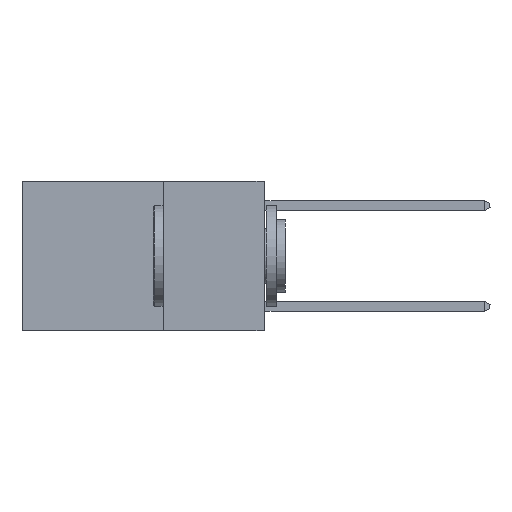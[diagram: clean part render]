
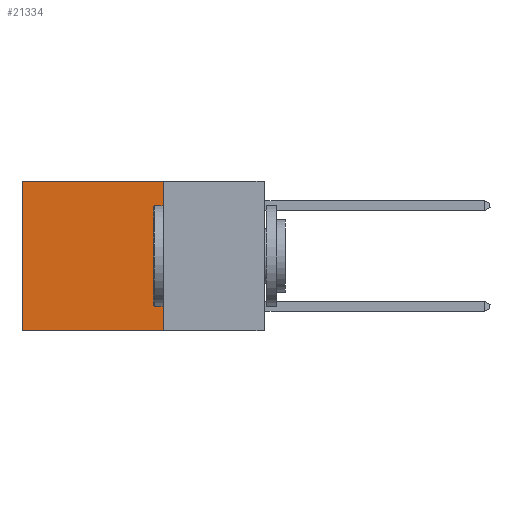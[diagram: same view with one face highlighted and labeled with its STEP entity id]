
A CAD part, left-side view. The second image highlights one B-rep face of the part: STEP entity #21334.
In plain terms, the highlighted planar face has unit normal (-1, 0, 0).
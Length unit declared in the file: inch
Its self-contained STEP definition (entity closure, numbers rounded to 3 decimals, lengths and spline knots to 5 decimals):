
#48 = CARTESIAN_POINT ( 'NONE',  ( 0.2625, 0.25, 0. ) ) ;
#140 = ORIENTED_EDGE ( 'NONE', *, *, #26880, .F. ) ;
#2336 = ORIENTED_EDGE ( 'NONE', *, *, #18239, .T. ) ;
#4314 = LINE ( 'NONE', #48, #22422 ) ;
#4949 = AXIS2_PLACEMENT_3D ( 'NONE', #7868, #18601, #25363 ) ;
#5242 = VERTEX_POINT ( 'NONE', #26752 ) ;
#5942 = CARTESIAN_POINT ( 'NONE',  ( 0.2625, 0.25, -0.37 ) ) ;
#6466 = CARTESIAN_POINT ( 'NONE',  ( 0.2625, 0.6, 0. ) ) ;
#7041 = DIRECTION ( 'NONE',  ( 0., 0., -1. ) ) ;
#7868 = CARTESIAN_POINT ( 'NONE',  ( 0.2625, 0.25, 0. ) ) ;
#8757 = CARTESIAN_POINT ( 'NONE',  ( 0.2625, 0.25, 0. ) ) ;
#8988 = CARTESIAN_POINT ( 'NONE',  ( 0.2625, 0.25, 0. ) ) ;
#9636 = ORIENTED_EDGE ( 'NONE', *, *, #13031, .T. ) ;
#10252 = VERTEX_POINT ( 'NONE', #8988 ) ;
#13031 = EDGE_CURVE ( 'NONE', #10252, #25060, #4314, .T. ) ;
#14917 = DIRECTION ( 'NONE',  ( 0., 1., 0. ) ) ;
#16838 = FACE_OUTER_BOUND ( 'NONE', #17917, .T. ) ;
#17717 = VECTOR ( 'NONE', #21857, 39.37008 ) ;
#17917 = EDGE_LOOP ( 'NONE', ( #2336, #140, #21682, #9636 ) ) ;
#18239 = EDGE_CURVE ( 'NONE', #25060, #28006, #26602, .T. ) ;
#18601 = DIRECTION ( 'NONE',  ( 1., 0., 0. ) ) ;
#19354 = LINE ( 'NONE', #8757, #17717 ) ;
#21334 = ADVANCED_FACE ( 'NONE', ( #16838 ), #27427, .F. ) ;
#21682 = ORIENTED_EDGE ( 'NONE', *, *, #23114, .F. ) ;
#21857 = DIRECTION ( 'NONE',  ( 0., 0., -1. ) ) ;
#22422 = VECTOR ( 'NONE', #28882, 39.37008 ) ;
#22935 = VECTOR ( 'NONE', #14917, 39.37008 ) ;
#23114 = EDGE_CURVE ( 'NONE', #10252, #5242, #19354, .T. ) ;
#23870 = LINE ( 'NONE', #5942, #22935 ) ;
#24600 = CARTESIAN_POINT ( 'NONE',  ( 0.2625, 0.6, 0. ) ) ;
#25060 = VERTEX_POINT ( 'NONE', #24600 ) ;
#25363 = DIRECTION ( 'NONE',  ( 0., 0., -1. ) ) ;
#25451 = CARTESIAN_POINT ( 'NONE',  ( 0.2625, 0.6, -0.37 ) ) ;
#26602 = LINE ( 'NONE', #6466, #28782 ) ;
#26752 = CARTESIAN_POINT ( 'NONE',  ( 0.2625, 0.25, -0.37 ) ) ;
#26880 = EDGE_CURVE ( 'NONE', #5242, #28006, #23870, .T. ) ;
#27427 = PLANE ( 'NONE',  #4949 ) ;
#28006 = VERTEX_POINT ( 'NONE', #25451 ) ;
#28782 = VECTOR ( 'NONE', #7041, 39.37008 ) ;
#28882 = DIRECTION ( 'NONE',  ( 0., 1., 0. ) ) ;
